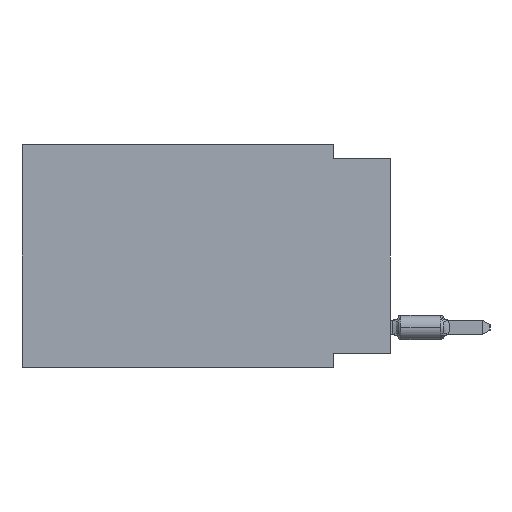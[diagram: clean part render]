
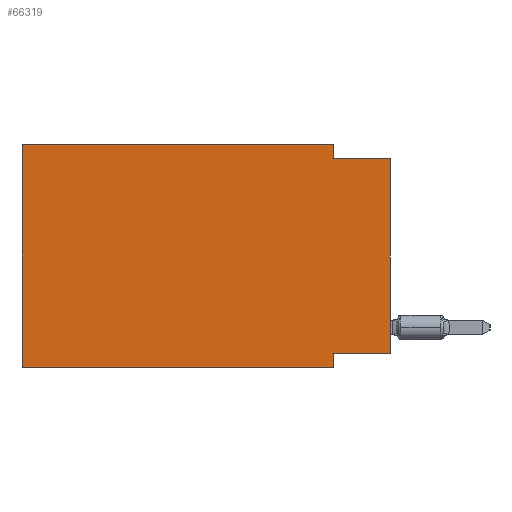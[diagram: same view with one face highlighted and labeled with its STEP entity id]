
A CAD part, left-side view. The second image highlights one B-rep face of the part: STEP entity #66319.
In plain terms, the highlighted planar face has unit normal (-1, 0, 0).
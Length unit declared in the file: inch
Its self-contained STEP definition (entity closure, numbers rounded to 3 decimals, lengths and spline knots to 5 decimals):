
#386 = DIRECTION ( 'NONE',  ( 0., -1., 0. ) ) ;
#1520 = VERTEX_POINT ( 'NONE', #34165 ) ;
#2677 = VERTEX_POINT ( 'NONE', #84842 ) ;
#4147 = VECTOR ( 'NONE', #33117, 39.37008 ) ;
#4417 = ORIENTED_EDGE ( 'NONE', *, *, #25275, .F. ) ;
#5939 = LINE ( 'NONE', #26445, #4147 ) ;
#8715 = VERTEX_POINT ( 'NONE', #31741 ) ;
#9910 = VECTOR ( 'NONE', #26305, 39.37008 ) ;
#10807 = CARTESIAN_POINT ( 'NONE',  ( 0., 0.1, -0.39 ) ) ;
#11257 = DIRECTION ( 'NONE',  ( 0., -1., 0. ) ) ;
#11502 = CARTESIAN_POINT ( 'NONE',  ( 0., 0.1, -0.39 ) ) ;
#12381 = VECTOR ( 'NONE', #24183, 39.37008 ) ;
#13378 = LINE ( 'NONE', #46783, #9910 ) ;
#14021 = EDGE_LOOP ( 'NONE', ( #42640, #42783, #4417, #38597, #71348, #86281, #20141, #56122 ) ) ;
#15536 = VERTEX_POINT ( 'NONE', #11502 ) ;
#16427 = AXIS2_PLACEMENT_3D ( 'NONE', #39734, #31753, #79420 ) ;
#17684 = CARTESIAN_POINT ( 'NONE',  ( 0., 0.645, -0.39 ) ) ;
#20141 = ORIENTED_EDGE ( 'NONE', *, *, #35574, .F. ) ;
#24183 = DIRECTION ( 'NONE',  ( 0., 0., 1. ) ) ;
#24878 = EDGE_CURVE ( 'NONE', #85466, #1520, #36301, .T. ) ;
#25275 = EDGE_CURVE ( 'NONE', #8715, #2677, #5939, .T. ) ;
#26305 = DIRECTION ( 'NONE',  ( 0., -1., 0. ) ) ;
#26445 = CARTESIAN_POINT ( 'NONE',  ( 0., 0.1, 0. ) ) ;
#30077 = CARTESIAN_POINT ( 'NONE',  ( 0., 0., -0.365 ) ) ;
#31429 = VERTEX_POINT ( 'NONE', #63200 ) ;
#31741 = CARTESIAN_POINT ( 'NONE',  ( 0., 0.1, 0. ) ) ;
#31753 = DIRECTION ( 'NONE',  ( 1., 0., 0. ) ) ;
#33117 = DIRECTION ( 'NONE',  ( 0., 0., -1. ) ) ;
#34165 = CARTESIAN_POINT ( 'NONE',  ( 0., 0.1, -0.365 ) ) ;
#35574 = EDGE_CURVE ( 'NONE', #1520, #15536, #86083, .T. ) ;
#36301 = LINE ( 'NONE', #30077, #66726 ) ;
#37991 = FACE_OUTER_BOUND ( 'NONE', #14021, .T. ) ;
#38597 = ORIENTED_EDGE ( 'NONE', *, *, #72632, .F. ) ;
#39734 = CARTESIAN_POINT ( 'NONE',  ( 0., 0.645, 0. ) ) ;
#40180 = LINE ( 'NONE', #79423, #72935 ) ;
#42513 = CARTESIAN_POINT ( 'NONE',  ( 0., 0., -0.365 ) ) ;
#42640 = ORIENTED_EDGE ( 'NONE', *, *, #49792, .T. ) ;
#42723 = CARTESIAN_POINT ( 'NONE',  ( 0., 0., 0. ) ) ;
#42783 = ORIENTED_EDGE ( 'NONE', *, *, #64138, .F. ) ;
#42984 = DIRECTION ( 'NONE',  ( 0., 1., 0. ) ) ;
#43911 = VERTEX_POINT ( 'NONE', #17684 ) ;
#45627 = VERTEX_POINT ( 'NONE', #66169 ) ;
#46783 = CARTESIAN_POINT ( 'NONE',  ( 0., 0.645, 0. ) ) ;
#49792 = EDGE_CURVE ( 'NONE', #85466, #45627, #55631, .T. ) ;
#55631 = LINE ( 'NONE', #42723, #79695 ) ;
#56122 = ORIENTED_EDGE ( 'NONE', *, *, #24878, .F. ) ;
#58021 = LINE ( 'NONE', #85215, #12381 ) ;
#61408 = CARTESIAN_POINT ( 'NONE',  ( 0., 0., -0.025 ) ) ;
#63200 = CARTESIAN_POINT ( 'NONE',  ( 0., 0.645, 0. ) ) ;
#63206 = DIRECTION ( 'NONE',  ( 0., 0., 1. ) ) ;
#64138 = EDGE_CURVE ( 'NONE', #2677, #45627, #68975, .T. ) ;
#65158 = DIRECTION ( 'NONE',  ( 0., 0., -1. ) ) ;
#66169 = CARTESIAN_POINT ( 'NONE',  ( 0., 0., -0.025 ) ) ;
#66319 = ADVANCED_FACE ( 'NONE', ( #37991 ), #86097, .F. ) ;
#66726 = VECTOR ( 'NONE', #42984, 39.37008 ) ;
#67651 = VECTOR ( 'NONE', #65158, 39.37008 ) ;
#68809 = VECTOR ( 'NONE', #386, 39.37008 ) ;
#68975 = LINE ( 'NONE', #61408, #68809 ) ;
#71348 = ORIENTED_EDGE ( 'NONE', *, *, #82195, .F. ) ;
#72632 = EDGE_CURVE ( 'NONE', #31429, #8715, #13378, .T. ) ;
#72935 = VECTOR ( 'NONE', #11257, 39.37008 ) ;
#75500 = EDGE_CURVE ( 'NONE', #43911, #15536, #40180, .T. ) ;
#79420 = DIRECTION ( 'NONE',  ( 0., 0., -1. ) ) ;
#79423 = CARTESIAN_POINT ( 'NONE',  ( 0., 0.645, -0.39 ) ) ;
#79695 = VECTOR ( 'NONE', #63206, 39.37008 ) ;
#82195 = EDGE_CURVE ( 'NONE', #43911, #31429, #58021, .T. ) ;
#84842 = CARTESIAN_POINT ( 'NONE',  ( 0., 0.1, -0.025 ) ) ;
#85215 = CARTESIAN_POINT ( 'NONE',  ( 0., 0.645, 0. ) ) ;
#85466 = VERTEX_POINT ( 'NONE', #42513 ) ;
#86083 = LINE ( 'NONE', #10807, #67651 ) ;
#86097 = PLANE ( 'NONE',  #16427 ) ;
#86281 = ORIENTED_EDGE ( 'NONE', *, *, #75500, .T. ) ;
